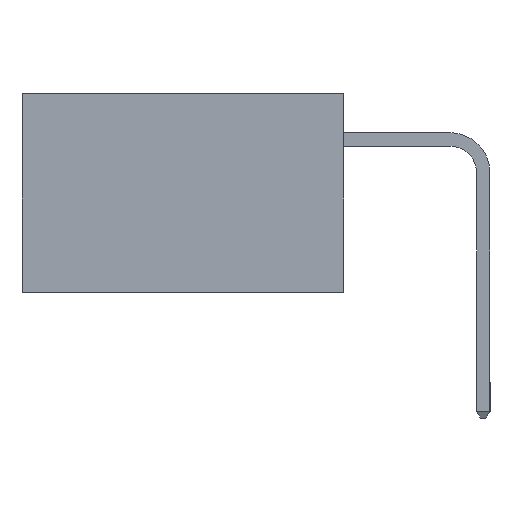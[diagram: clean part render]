
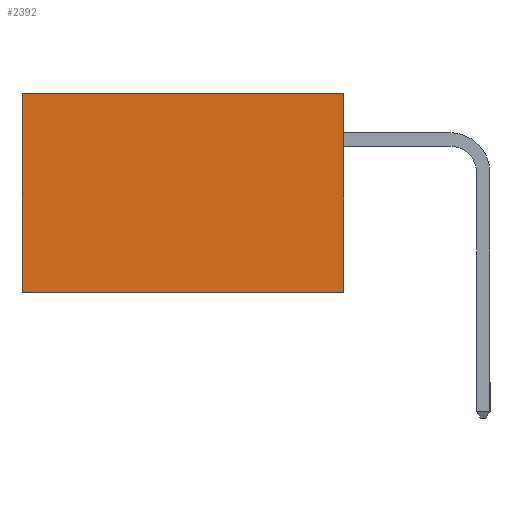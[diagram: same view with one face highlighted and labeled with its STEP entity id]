
A CAD part, left-side view. The second image highlights one B-rep face of the part: STEP entity #2392.
In plain terms, the highlighted planar face has unit normal (-1, 0, 0).
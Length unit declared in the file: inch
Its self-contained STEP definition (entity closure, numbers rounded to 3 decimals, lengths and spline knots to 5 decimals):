
#171 = ORIENTED_EDGE ( 'NONE', *, *, #901, .F. ) ;
#658 = DIRECTION ( 'NONE',  ( 0., 1., 0. ) ) ;
#669 = CARTESIAN_POINT ( 'NONE',  ( 0.298, 0., -0.37 ) ) ;
#901 = EDGE_CURVE ( 'NONE', #9794, #8932, #3199, .T. ) ;
#1276 = EDGE_CURVE ( 'NONE', #2149, #9964, #4272, .T. ) ;
#1440 = DIRECTION ( 'NONE',  ( 0., 0., -1. ) ) ;
#2149 = VERTEX_POINT ( 'NONE', #8846 ) ;
#2322 = LINE ( 'NONE', #669, #2869 ) ;
#2392 = ADVANCED_FACE ( 'NONE', ( #6098 ), #9724, .F. ) ;
#2474 = ORIENTED_EDGE ( 'NONE', *, *, #7247, .T. ) ;
#2869 = VECTOR ( 'NONE', #658, 39.37008 ) ;
#3199 = LINE ( 'NONE', #8527, #7452 ) ;
#3684 = LINE ( 'NONE', #7313, #10177 ) ;
#3942 = CARTESIAN_POINT ( 'NONE',  ( 0.298, 0., -0.37 ) ) ;
#4044 = DIRECTION ( 'NONE',  ( 0., 1., 0. ) ) ;
#4272 = LINE ( 'NONE', #7774, #8508 ) ;
#4467 = EDGE_LOOP ( 'NONE', ( #9936, #9666, #171, #2474 ) ) ;
#4657 = DIRECTION ( 'NONE',  ( 0., 0., -1. ) ) ;
#6098 = FACE_OUTER_BOUND ( 'NONE', #4467, .T. ) ;
#6472 = CARTESIAN_POINT ( 'NONE',  ( 0.298, 0., 0. ) ) ;
#6692 = EDGE_CURVE ( 'NONE', #8932, #9964, #2322, .T. ) ;
#6950 = DIRECTION ( 'NONE',  ( 0., 0., -1. ) ) ;
#7247 = EDGE_CURVE ( 'NONE', #9794, #2149, #3684, .T. ) ;
#7313 = CARTESIAN_POINT ( 'NONE',  ( 0.298, 0., 0. ) ) ;
#7452 = VECTOR ( 'NONE', #4657, 39.37008 ) ;
#7774 = CARTESIAN_POINT ( 'NONE',  ( 0.298, 0.6, 0. ) ) ;
#8358 = CARTESIAN_POINT ( 'NONE',  ( 0.298, 0.6, -0.37 ) ) ;
#8508 = VECTOR ( 'NONE', #1440, 39.37008 ) ;
#8527 = CARTESIAN_POINT ( 'NONE',  ( 0.298, 0., 0. ) ) ;
#8833 = AXIS2_PLACEMENT_3D ( 'NONE', #10027, #9737, #6950 ) ;
#8846 = CARTESIAN_POINT ( 'NONE',  ( 0.298, 0.6, 0. ) ) ;
#8932 = VERTEX_POINT ( 'NONE', #3942 ) ;
#9666 = ORIENTED_EDGE ( 'NONE', *, *, #6692, .F. ) ;
#9724 = PLANE ( 'NONE',  #8833 ) ;
#9737 = DIRECTION ( 'NONE',  ( 1., 0., 0. ) ) ;
#9794 = VERTEX_POINT ( 'NONE', #6472 ) ;
#9936 = ORIENTED_EDGE ( 'NONE', *, *, #1276, .T. ) ;
#9964 = VERTEX_POINT ( 'NONE', #8358 ) ;
#10027 = CARTESIAN_POINT ( 'NONE',  ( 0.298, 0., 0. ) ) ;
#10177 = VECTOR ( 'NONE', #4044, 39.37008 ) ;
